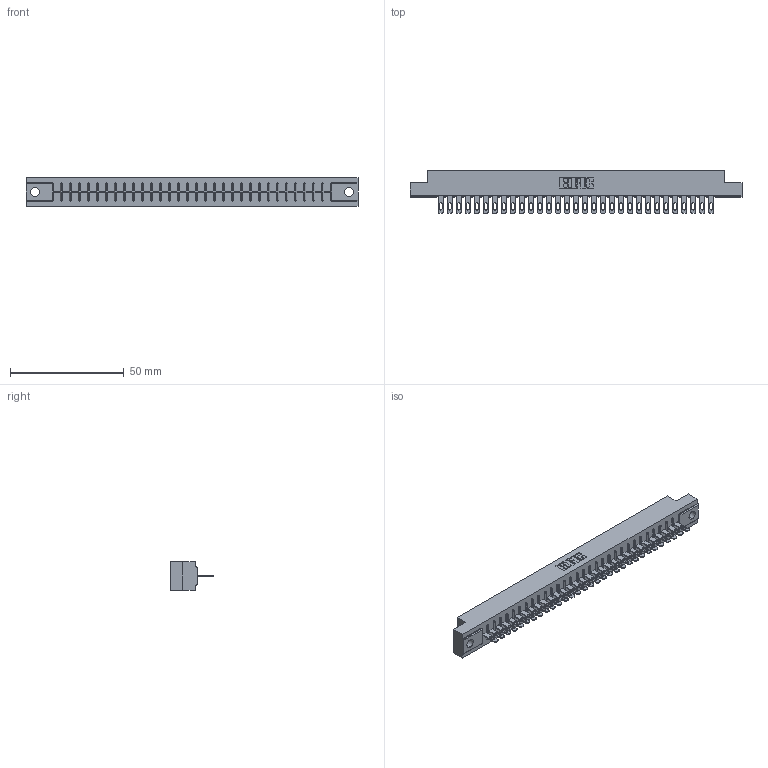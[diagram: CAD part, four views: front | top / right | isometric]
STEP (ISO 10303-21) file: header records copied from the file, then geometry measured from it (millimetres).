
FILE_DESCRIPTION (( 'STEP AP203' ), '1' );
FILE_NAME ('356-031-400-104.STEP', '2020-09-23T20:43:02', ( '' ), ( '' ), 'SwSTEP 2.0', 'SolidWorks 2020', '' );
FILE_SCHEMA (( 'CONFIG_CONTROL_DESIGN' ));
Length unit declared in the file: inch
Products named in the file (3): 356-031-400-104; 306 Part_.156 Dia; 306-290-001_100
Assembly tree (32 placements, depth 2):
  356-031-400-104
    306 Part_.156 Dia
    306-290-001_100  x31
Bounding box: 145.85 x 18.87 x 12.7 mm (x, y, z)
Volume: 16019.8 mm3; surface area: 16690.6 mm2
Topology: 32 solids, 32 shells, 2486 faces, 7017 edges, 4510 vertices
Faces by surface type: plane 1632, cylinder 730, sphere 124
Entity records: 30916 total; most frequent: CARTESIAN_POINT 5194, ORIENTED_EDGE 5146, DIRECTION 5115, EDGE_CURVE 2573, VECTOR 2013, LINE 2013, VERTEX_POINT 1630, AXIS2_PLACEMENT_3D 1551
